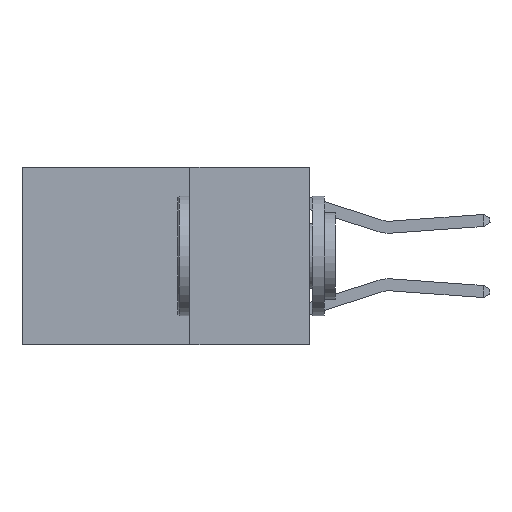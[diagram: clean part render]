
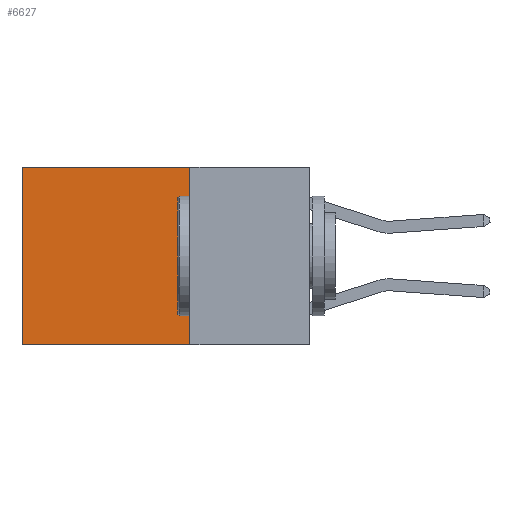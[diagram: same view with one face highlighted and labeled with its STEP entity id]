
A CAD part, left-side view. The second image highlights one B-rep face of the part: STEP entity #6627.
In plain terms, the highlighted planar face has unit normal (-1, 0, 0).
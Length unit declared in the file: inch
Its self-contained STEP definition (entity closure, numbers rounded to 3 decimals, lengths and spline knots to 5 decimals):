
#334 = CARTESIAN_POINT ( 'NONE',  ( 0.2625, 0.25, 0. ) ) ;
#454 = PLANE ( 'NONE',  #3801 ) ;
#499 = DIRECTION ( 'NONE',  ( 0., 0., -1. ) ) ;
#580 = CARTESIAN_POINT ( 'NONE',  ( 0.2625, 0.25, -0.37 ) ) ;
#1185 = FACE_OUTER_BOUND ( 'NONE', #7929, .T. ) ;
#1267 = DIRECTION ( 'NONE',  ( 0., 1., 0. ) ) ;
#1889 = DIRECTION ( 'NONE',  ( 1., 0., 0. ) ) ;
#1945 = CARTESIAN_POINT ( 'NONE',  ( 0.2625, 0.25, 0. ) ) ;
#2117 = EDGE_CURVE ( 'NONE', #9294, #3371, #6047, .T. ) ;
#2147 = CARTESIAN_POINT ( 'NONE',  ( 0.2625, 0.6, 0. ) ) ;
#2353 = ORIENTED_EDGE ( 'NONE', *, *, #4863, .F. ) ;
#2472 = CARTESIAN_POINT ( 'NONE',  ( 0.2625, 0.6, 0. ) ) ;
#3371 = VERTEX_POINT ( 'NONE', #9331 ) ;
#3801 = AXIS2_PLACEMENT_3D ( 'NONE', #1945, #1889, #8749 ) ;
#4248 = DIRECTION ( 'NONE',  ( 0., 1., 0. ) ) ;
#4461 = ORIENTED_EDGE ( 'NONE', *, *, #2117, .T. ) ;
#4863 = EDGE_CURVE ( 'NONE', #7791, #3371, #9730, .T. ) ;
#4998 = VERTEX_POINT ( 'NONE', #8939 ) ;
#6047 = LINE ( 'NONE', #2472, #10088 ) ;
#6102 = LINE ( 'NONE', #10093, #8087 ) ;
#6287 = CARTESIAN_POINT ( 'NONE',  ( 0.2625, 0.25, -0.37 ) ) ;
#6627 = ADVANCED_FACE ( 'NONE', ( #1185 ), #454, .F. ) ;
#7791 = VERTEX_POINT ( 'NONE', #580 ) ;
#7929 = EDGE_LOOP ( 'NONE', ( #4461, #2353, #10060, #10101 ) ) ;
#8087 = VECTOR ( 'NONE', #4248, 39.37008 ) ;
#8749 = DIRECTION ( 'NONE',  ( 0., 0., -1. ) ) ;
#8939 = CARTESIAN_POINT ( 'NONE',  ( 0.2625, 0.25, 0. ) ) ;
#9278 = DIRECTION ( 'NONE',  ( 0., 0., -1. ) ) ;
#9294 = VERTEX_POINT ( 'NONE', #2147 ) ;
#9331 = CARTESIAN_POINT ( 'NONE',  ( 0.2625, 0.6, -0.37 ) ) ;
#9683 = LINE ( 'NONE', #334, #10126 ) ;
#9730 = LINE ( 'NONE', #6287, #10352 ) ;
#9790 = EDGE_CURVE ( 'NONE', #4998, #7791, #9683, .T. ) ;
#10017 = EDGE_CURVE ( 'NONE', #4998, #9294, #6102, .T. ) ;
#10060 = ORIENTED_EDGE ( 'NONE', *, *, #9790, .F. ) ;
#10088 = VECTOR ( 'NONE', #9278, 39.37008 ) ;
#10093 = CARTESIAN_POINT ( 'NONE',  ( 0.2625, 0.25, 0. ) ) ;
#10101 = ORIENTED_EDGE ( 'NONE', *, *, #10017, .T. ) ;
#10126 = VECTOR ( 'NONE', #499, 39.37008 ) ;
#10352 = VECTOR ( 'NONE', #1267, 39.37008 ) ;
